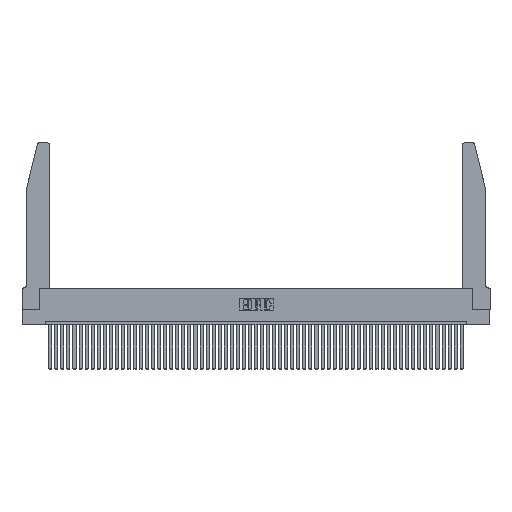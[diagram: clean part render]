
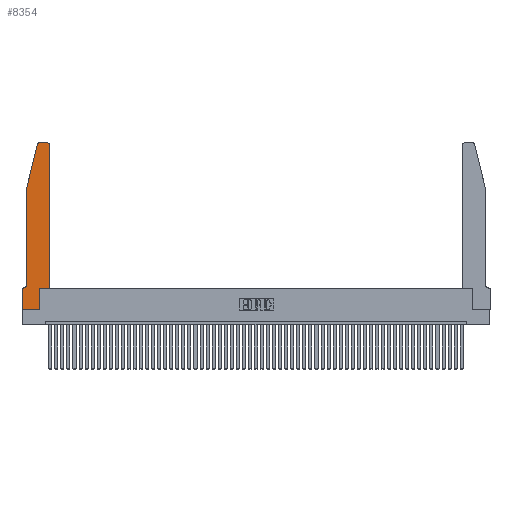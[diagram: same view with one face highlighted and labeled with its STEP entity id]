
A CAD part, top view. The second image highlights one B-rep face of the part: STEP entity #8354.
In plain terms, the highlighted planar face has unit normal (0, 0, 1).
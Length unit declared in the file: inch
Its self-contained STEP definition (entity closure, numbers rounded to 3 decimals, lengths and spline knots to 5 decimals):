
#848 = EDGE_CURVE ( 'NONE', #33379, #25439, #9719, .T. ) ;
#1833 = VECTOR ( 'NONE', #42197, 39.37008 ) ;
#2042 = ORIENTED_EDGE ( 'NONE', *, *, #27168, .T. ) ;
#3105 = DIRECTION ( 'NONE',  ( 0., 0., -1. ) ) ;
#3647 = DIRECTION ( 'NONE',  ( 0., -1., 0. ) ) ;
#3845 = AXIS2_PLACEMENT_3D ( 'NONE', #43165, #15043, #52304 ) ;
#4379 = CARTESIAN_POINT ( 'NONE',  ( 0.4505, 2.72, 0.37 ) ) ;
#5072 = VERTEX_POINT ( 'NONE', #45045 ) ;
#5406 = DIRECTION ( 'NONE',  ( 1., 0., 0. ) ) ;
#5648 = CARTESIAN_POINT ( 'NONE',  ( 0., 0., 0.37 ) ) ;
#5996 = AXIS2_PLACEMENT_3D ( 'NONE', #22809, #9937, #42487 ) ;
#6754 = EDGE_CURVE ( 'NONE', #33092, #51658, #35679, .T. ) ;
#6906 = CARTESIAN_POINT ( 'NONE',  ( 0.4505, 0.35, 0.37 ) ) ;
#7072 = VERTEX_POINT ( 'NONE', #11463 ) ;
#7147 = LINE ( 'NONE', #21574, #1833 ) ;
#7307 = VERTEX_POINT ( 'NONE', #47713 ) ;
#7873 = ORIENTED_EDGE ( 'NONE', *, *, #6754, .T. ) ;
#8354 = ADVANCED_FACE ( 'NONE', ( #46198 ), #33572, .T. ) ;
#8768 = EDGE_CURVE ( 'NONE', #22159, #41964, #48261, .T. ) ;
#9407 = VERTEX_POINT ( 'NONE', #20698 ) ;
#9719 = CIRCLE ( 'NONE', #5996, 0.03 ) ;
#9937 = DIRECTION ( 'NONE',  ( 0., 0., 1. ) ) ;
#9969 = CARTESIAN_POINT ( 'NONE',  ( 0.284, 2.75, 0.37 ) ) ;
#11463 = CARTESIAN_POINT ( 'NONE',  ( 0.2865, 0., 0.37 ) ) ;
#13440 = CARTESIAN_POINT ( 'NONE',  ( 0.4505, 0.35, 0.37 ) ) ;
#14810 = ORIENTED_EDGE ( 'NONE', *, *, #26912, .T. ) ;
#15043 = DIRECTION ( 'NONE',  ( 0., 0., 1. ) ) ;
#15358 = DIRECTION ( 'NONE',  ( -1., 0., 0. ) ) ;
#15819 = VECTOR ( 'NONE', #44342, 39.37008 ) ;
#16182 = CARTESIAN_POINT ( 'NONE',  ( 0.4205, 2.75, 0.37 ) ) ;
#16605 = EDGE_CURVE ( 'NONE', #45004, #33379, #40559, .T. ) ;
#16932 = ORIENTED_EDGE ( 'NONE', *, *, #16605, .T. ) ;
#17069 = CARTESIAN_POINT ( 'NONE',  ( 0.0755, 0.35, 0.37 ) ) ;
#17540 = DIRECTION ( 'NONE',  ( 0., 0., 1. ) ) ;
#17926 = ORIENTED_EDGE ( 'NONE', *, *, #848, .T. ) ;
#18068 = CARTESIAN_POINT ( 'NONE',  ( 0.0055, 0.35, 0.37 ) ) ;
#18883 = LINE ( 'NONE', #5648, #49967 ) ;
#19779 = DIRECTION ( 'NONE',  ( 1., 0., 0. ) ) ;
#19903 = DIRECTION ( 'NONE',  ( -1., 0., 0. ) ) ;
#20698 = CARTESIAN_POINT ( 'NONE',  ( 0.2865, 0.35, 0.37 ) ) ;
#20790 = EDGE_CURVE ( 'NONE', #7072, #9407, #34969, .T. ) ;
#21539 = VECTOR ( 'NONE', #3647, 39.37008 ) ;
#21574 = CARTESIAN_POINT ( 'NONE',  ( 0., 0., 0.37 ) ) ;
#22004 = CARTESIAN_POINT ( 'NONE',  ( 0.2605, 2.75, 0.37 ) ) ;
#22159 = VERTEX_POINT ( 'NONE', #37434 ) ;
#22452 = VERTEX_POINT ( 'NONE', #9969 ) ;
#22681 = EDGE_CURVE ( 'NONE', #7307, #5072, #18883, .T. ) ;
#22809 = CARTESIAN_POINT ( 'NONE',  ( 0.4205, 2.72, 0.37 ) ) ;
#23549 = CIRCLE ( 'NONE', #3845, 0.03 ) ;
#24112 = AXIS2_PLACEMENT_3D ( 'NONE', #27768, #3105, #19903 ) ;
#24234 = VECTOR ( 'NONE', #30512, 39.37008 ) ;
#25439 = VERTEX_POINT ( 'NONE', #16182 ) ;
#25864 = CARTESIAN_POINT ( 'NONE',  ( 0.2865, 0.35, 0.37 ) ) ;
#26912 = EDGE_CURVE ( 'NONE', #41964, #33092, #38776, .T. ) ;
#27168 = EDGE_CURVE ( 'NONE', #22452, #22159, #23549, .T. ) ;
#27768 = CARTESIAN_POINT ( 'NONE',  ( 0.0055, 0.42, 0.37 ) ) ;
#28872 = DIRECTION ( 'NONE',  ( -1., 0., 0. ) ) ;
#28993 = ORIENTED_EDGE ( 'NONE', *, *, #52434, .T. ) ;
#29109 = ORIENTED_EDGE ( 'NONE', *, *, #50735, .T. ) ;
#29386 = DIRECTION ( 'NONE',  ( 0., -1., 0. ) ) ;
#29814 = AXIS2_PLACEMENT_3D ( 'NONE', #41894, #17540, #5406 ) ;
#30210 = EDGE_LOOP ( 'NONE', ( #39366, #2042, #52452, #14810, #7873, #29109, #52197, #28993, #51539, #38455, #16932, #17926 ) ) ;
#30512 = DIRECTION ( 'NONE',  ( 0., 1., 0. ) ) ;
#31482 = CARTESIAN_POINT ( 'NONE',  ( 0.0755, 2., 0.37 ) ) ;
#31552 = VECTOR ( 'NONE', #15358, 39.37008 ) ;
#32607 = CARTESIAN_POINT ( 'NONE',  ( 0.0755, 2., 0.37 ) ) ;
#33092 = VERTEX_POINT ( 'NONE', #38062 ) ;
#33129 = DIRECTION ( 'NONE',  ( 0., 1., 0. ) ) ;
#33379 = VERTEX_POINT ( 'NONE', #4379 ) ;
#33572 = PLANE ( 'NONE',  #29814 ) ;
#33853 = EDGE_CURVE ( 'NONE', #9407, #45004, #52674, .T. ) ;
#34110 = VECTOR ( 'NONE', #33129, 39.37008 ) ;
#34969 = LINE ( 'NONE', #25864, #24234 ) ;
#35679 = CIRCLE ( 'NONE', #24112, 0.07 ) ;
#37434 = CARTESIAN_POINT ( 'NONE',  ( 0.25487, 2.72718, 0.37 ) ) ;
#37846 = VECTOR ( 'NONE', #28872, 39.37008 ) ;
#38062 = CARTESIAN_POINT ( 'NONE',  ( 0.0755, 0.42, 0.37 ) ) ;
#38455 = ORIENTED_EDGE ( 'NONE', *, *, #33853, .T. ) ;
#38776 = LINE ( 'NONE', #40494, #21539 ) ;
#39218 = VECTOR ( 'NONE', #19779, 39.37008 ) ;
#39366 = ORIENTED_EDGE ( 'NONE', *, *, #51053, .T. ) ;
#40494 = CARTESIAN_POINT ( 'NONE',  ( 0.0755, 2., 0.37 ) ) ;
#40559 = LINE ( 'NONE', #13440, #34110 ) ;
#41894 = CARTESIAN_POINT ( 'NONE',  ( 0., 0.35, 0.37 ) ) ;
#41964 = VERTEX_POINT ( 'NONE', #31482 ) ;
#42197 = DIRECTION ( 'NONE',  ( 1., 0., 0. ) ) ;
#42487 = DIRECTION ( 'NONE',  ( 1., 0., 0. ) ) ;
#43165 = CARTESIAN_POINT ( 'NONE',  ( 0.284, 2.72, 0.37 ) ) ;
#44342 = DIRECTION ( 'NONE',  ( -0.239, -0.971, 0. ) ) ;
#44892 = LINE ( 'NONE', #17069, #37846 ) ;
#45004 = VERTEX_POINT ( 'NONE', #6906 ) ;
#45045 = CARTESIAN_POINT ( 'NONE',  ( 0., 0., 0.37 ) ) ;
#46198 = FACE_OUTER_BOUND ( 'NONE', #30210, .T. ) ;
#46762 = LINE ( 'NONE', #22004, #31552 ) ;
#47713 = CARTESIAN_POINT ( 'NONE',  ( 0., 0.35, 0.37 ) ) ;
#48261 = LINE ( 'NONE', #32607, #15819 ) ;
#49600 = CARTESIAN_POINT ( 'NONE',  ( 0.4505, 0.35, 0.37 ) ) ;
#49967 = VECTOR ( 'NONE', #29386, 39.37008 ) ;
#50735 = EDGE_CURVE ( 'NONE', #51658, #7307, #44892, .T. ) ;
#51053 = EDGE_CURVE ( 'NONE', #25439, #22452, #46762, .T. ) ;
#51539 = ORIENTED_EDGE ( 'NONE', *, *, #20790, .T. ) ;
#51658 = VERTEX_POINT ( 'NONE', #18068 ) ;
#52197 = ORIENTED_EDGE ( 'NONE', *, *, #22681, .T. ) ;
#52304 = DIRECTION ( 'NONE',  ( 1., 0., 0. ) ) ;
#52434 = EDGE_CURVE ( 'NONE', #5072, #7072, #7147, .T. ) ;
#52452 = ORIENTED_EDGE ( 'NONE', *, *, #8768, .T. ) ;
#52674 = LINE ( 'NONE', #49600, #39218 ) ;
